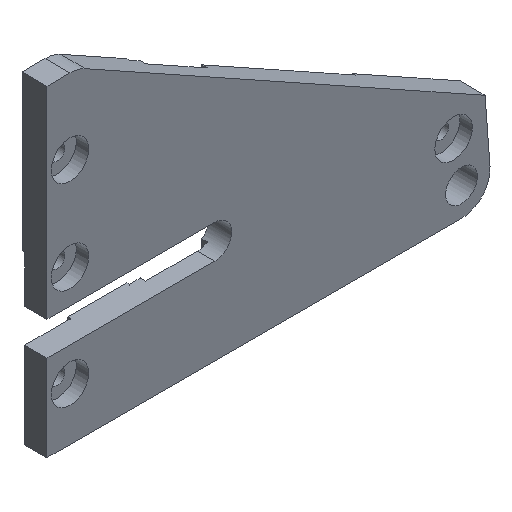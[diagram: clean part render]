
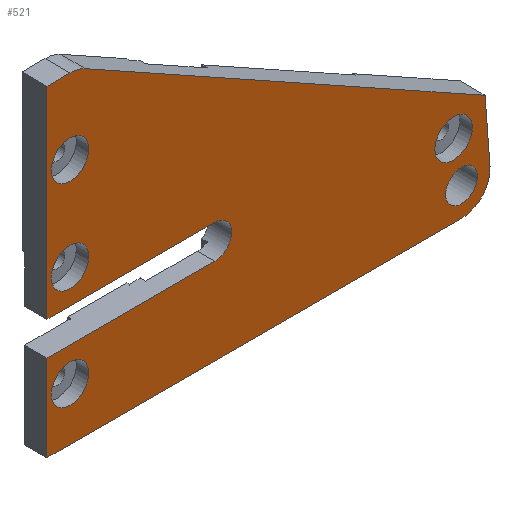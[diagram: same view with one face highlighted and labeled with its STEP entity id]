
A CAD part, isometric view. The second image highlights one B-rep face of the part: STEP entity #521.
In plain terms, the highlighted planar face has unit normal (0, -1, 0).
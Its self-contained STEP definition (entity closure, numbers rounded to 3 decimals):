
#18 = ORIENTED_EDGE ( 'NONE', *, *, #1301, .T. ) ;
#49 = EDGE_CURVE ( 'NONE', #352, #352, #270, .T. ) ;
#84 = EDGE_CURVE ( 'NONE', #267, #700, #531, .T. ) ;
#111 = CARTESIAN_POINT ( 'NONE',  ( 4.597, -5., -33.63 ) ) ;
#112 = EDGE_LOOP ( 'NONE', ( #823 ) ) ;
#125 = ORIENTED_EDGE ( 'NONE', *, *, #84, .T. ) ;
#140 = DIRECTION ( 'NONE',  ( 0., -1., 0. ) ) ;
#162 = CARTESIAN_POINT ( 'NONE',  ( 0., -5., 0. ) ) ;
#174 = FACE_BOUND ( 'NONE', #292, .T. ) ;
#187 = LINE ( 'NONE', #744, #439 ) ;
#190 = VECTOR ( 'NONE', #1303, 1000. ) ;
#191 = VERTEX_POINT ( 'NONE', #162 ) ;
#199 = CARTESIAN_POINT ( 'NONE',  ( 4.597, -5., -57.573 ) ) ;
#203 = VERTEX_POINT ( 'NONE', #1128 ) ;
#210 = CARTESIAN_POINT ( 'NONE',  ( 33.579, -5., -43.726 ) ) ;
#220 = DIRECTION ( 'NONE',  ( 0., 0., -1. ) ) ;
#244 = ORIENTED_EDGE ( 'NONE', *, *, #445, .T. ) ;
#247 = ORIENTED_EDGE ( 'NONE', *, *, #398, .F. ) ;
#254 = VERTEX_POINT ( 'NONE', #737 ) ;
#258 = CARTESIAN_POINT ( 'NONE',  ( 81.344, -5., -49.72 ) ) ;
#260 = LINE ( 'NONE', #1119, #1366 ) ;
#267 = VERTEX_POINT ( 'NONE', #607 ) ;
#270 = CIRCLE ( 'NONE', #540, 3.75 ) ;
#279 = EDGE_CURVE ( 'NONE', #687, #1189, #896, .T. ) ;
#289 = VERTEX_POINT ( 'NONE', #1157 ) ;
#292 = EDGE_LOOP ( 'NONE', ( #1288 ) ) ;
#303 = CARTESIAN_POINT ( 'NONE',  ( 82.931, -5., -55.474 ) ) ;
#317 = AXIS2_PLACEMENT_3D ( 'NONE', #1224, #589, #1336 ) ;
#320 = DIRECTION ( 'NONE',  ( 0., 0., 1. ) ) ;
#324 = EDGE_CURVE ( 'NONE', #1141, #1141, #838, .T. ) ;
#328 = CARTESIAN_POINT ( 'NONE',  ( 0., -5., 0. ) ) ;
#330 = LINE ( 'NONE', #328, #1144 ) ;
#337 = AXIS2_PLACEMENT_3D ( 'NONE', #983, #345, #1096 ) ;
#343 = CIRCLE ( 'NONE', #1369, 3.366 ) ;
#345 = DIRECTION ( 'NONE',  ( 0., -1., 0. ) ) ;
#352 = VERTEX_POINT ( 'NONE', #622 ) ;
#355 = DIRECTION ( 'NONE',  ( 0., 1., 0. ) ) ;
#357 = CIRCLE ( 'NONE', #966, 3.75 ) ;
#359 = AXIS2_PLACEMENT_3D ( 'NONE', #614, #1357, #721 ) ;
#361 = DIRECTION ( 'NONE',  ( 0., 0., -1. ) ) ;
#384 = CARTESIAN_POINT ( 'NONE',  ( 1.482, -5., 2.657 ) ) ;
#391 = DIRECTION ( 'NONE',  ( 1., 0., 0. ) ) ;
#398 = EDGE_CURVE ( 'NONE', #584, #203, #343, .T. ) ;
#402 = ORIENTED_EDGE ( 'NONE', *, *, #279, .T. ) ;
#415 = LINE ( 'NONE', #613, #947 ) ;
#426 = LINE ( 'NONE', #1245, #1237 ) ;
#427 = VERTEX_POINT ( 'NONE', #1196 ) ;
#432 = DIRECTION ( 'NONE',  ( 0., 0., -1. ) ) ;
#439 = VECTOR ( 'NONE', #1058, 1000. ) ;
#445 = EDGE_CURVE ( 'NONE', #700, #1307, #565, .T. ) ;
#455 = EDGE_LOOP ( 'NONE', ( #711 ) ) ;
#457 = CARTESIAN_POINT ( 'NONE',  ( 0., -5., 0. ) ) ;
#459 = FACE_BOUND ( 'NONE', #112, .T. ) ;
#474 = LINE ( 'NONE', #1193, #190 ) ;
#496 = DIRECTION ( 'NONE',  ( -0.873, 0., 0.487 ) ) ;
#514 = ORIENTED_EDGE ( 'NONE', *, *, #761, .F. ) ;
#521 = ADVANCED_FACE ( 'NONE', ( #459, #1311, #174, #1282, #991, #715 ), #992, .F. ) ;
#531 = LINE ( 'NONE', #900, #1025 ) ;
#540 = AXIS2_PLACEMENT_3D ( 'NONE', #787, #140, #894 ) ;
#565 = CIRCLE ( 'NONE', #337, 5.715 ) ;
#581 = CARTESIAN_POINT ( 'NONE',  ( 4.597, -5., 0. ) ) ;
#582 = EDGE_CURVE ( 'NONE', #289, #289, #357, .T. ) ;
#584 = VERTEX_POINT ( 'NONE', #791 ) ;
#589 = DIRECTION ( 'NONE',  ( 0., -1., 0. ) ) ;
#607 = CARTESIAN_POINT ( 'NONE',  ( 0., -5., -64.364 ) ) ;
#613 = CARTESIAN_POINT ( 'NONE',  ( 0., -5., -47.092 ) ) ;
#614 = CARTESIAN_POINT ( 'NONE',  ( 4.597, -5., -6.35 ) ) ;
#622 = CARTESIAN_POINT ( 'NONE',  ( 4.597, -5., -18.75 ) ) ;
#625 = CARTESIAN_POINT ( 'NONE',  ( 82.931, -5., -58.649 ) ) ;
#644 = EDGE_CURVE ( 'NONE', #191, #1189, #260, .T. ) ;
#653 = AXIS2_PLACEMENT_3D ( 'NONE', #625, #1370, #735 ) ;
#685 = DIRECTION ( 'NONE',  ( 1., 0., 0. ) ) ;
#687 = VERTEX_POINT ( 'NONE', #1343 ) ;
#700 = VERTEX_POINT ( 'NONE', #1127 ) ;
#711 = ORIENTED_EDGE ( 'NONE', *, *, #1235, .F. ) ;
#715 = FACE_OUTER_BOUND ( 'NONE', #745, .T. ) ;
#721 = DIRECTION ( 'NONE',  ( 0., 0., -1. ) ) ;
#735 = DIRECTION ( 'NONE',  ( 0., 0., 1. ) ) ;
#737 = CARTESIAN_POINT ( 'NONE',  ( 4.597, -5., -37.38 ) ) ;
#744 = CARTESIAN_POINT ( 'NONE',  ( 83.678, -5., 6.412 ) ) ;
#745 = EDGE_LOOP ( 'NONE', ( #402, #1186, #1165, #1176, #247, #514, #905, #125, #244, #1361, #18 ) ) ;
#761 = EDGE_CURVE ( 'NONE', #427, #584, #415, .T. ) ;
#787 = CARTESIAN_POINT ( 'NONE',  ( 4.597, -5., -15. ) ) ;
#789 = VERTEX_POINT ( 'NONE', #199 ) ;
#791 = CARTESIAN_POINT ( 'NONE',  ( 33.579, -5., -47.092 ) ) ;
#810 = LINE ( 'NONE', #384, #1344 ) ;
#823 = ORIENTED_EDGE ( 'NONE', *, *, #324, .T. ) ;
#838 = CIRCLE ( 'NONE', #653, 3.175 ) ;
#865 = DIRECTION ( 'NONE',  ( 0., -1., 0. ) ) ;
#873 = EDGE_CURVE ( 'NONE', #972, #1307, #187, .T. ) ;
#877 = CIRCLE ( 'NONE', #317, 3.75 ) ;
#893 = AXIS2_PLACEMENT_3D ( 'NONE', #457, #355, #1103 ) ;
#894 = DIRECTION ( 'NONE',  ( 0., 0., -1. ) ) ;
#896 = CIRCLE ( 'NONE', #359, 6.35 ) ;
#900 = CARTESIAN_POINT ( 'NONE',  ( 0., -5., -64.364 ) ) ;
#901 = ORIENTED_EDGE ( 'NONE', *, *, #582, .F. ) ;
#905 = ORIENTED_EDGE ( 'NONE', *, *, #1116, .T. ) ;
#906 = DIRECTION ( 'NONE',  ( 1., 0., 0. ) ) ;
#947 = VECTOR ( 'NONE', #391, 1000. ) ;
#956 = DIRECTION ( 'NONE',  ( 0., -1., 0. ) ) ;
#966 = AXIS2_PLACEMENT_3D ( 'NONE', #258, #1001, #361 ) ;
#972 = VERTEX_POINT ( 'NONE', #1283 ) ;
#983 = CARTESIAN_POINT ( 'NONE',  ( 82.931, -5., -58.649 ) ) ;
#991 = FACE_BOUND ( 'NONE', #455, .T. ) ;
#992 = PLANE ( 'NONE',  #893 ) ;
#994 = EDGE_CURVE ( 'NONE', #191, #1289, #330, .T. ) ;
#1001 = DIRECTION ( 'NONE',  ( 0., -1., 0. ) ) ;
#1010 = EDGE_CURVE ( 'NONE', #254, #254, #1180, .T. ) ;
#1025 = VECTOR ( 'NONE', #685, 1000. ) ;
#1040 = DIRECTION ( 'NONE',  ( -1., 0., 0. ) ) ;
#1049 = ORIENTED_EDGE ( 'NONE', *, *, #49, .F. ) ;
#1058 = DIRECTION ( 'NONE',  ( 0.076, 0., -0.997 ) ) ;
#1096 = DIRECTION ( 'NONE',  ( 0., 0., 1. ) ) ;
#1103 = DIRECTION ( 'NONE',  ( 0., 0., 1. ) ) ;
#1116 = EDGE_CURVE ( 'NONE', #427, #267, #474, .T. ) ;
#1119 = CARTESIAN_POINT ( 'NONE',  ( 0., -5., 0. ) ) ;
#1127 = CARTESIAN_POINT ( 'NONE',  ( 82.931, -5., -64.364 ) ) ;
#1128 = CARTESIAN_POINT ( 'NONE',  ( 33.579, -5., -40.361 ) ) ;
#1133 = CARTESIAN_POINT ( 'NONE',  ( 88.629, -5., -58.212 ) ) ;
#1141 = VERTEX_POINT ( 'NONE', #303 ) ;
#1144 = VECTOR ( 'NONE', #432, 1000. ) ;
#1157 = CARTESIAN_POINT ( 'NONE',  ( 81.344, -5., -53.47 ) ) ;
#1165 = ORIENTED_EDGE ( 'NONE', *, *, #994, .T. ) ;
#1176 = ORIENTED_EDGE ( 'NONE', *, *, #1355, .F. ) ;
#1180 = CIRCLE ( 'NONE', #1371, 3.75 ) ;
#1186 = ORIENTED_EDGE ( 'NONE', *, *, #644, .F. ) ;
#1189 = VERTEX_POINT ( 'NONE', #581 ) ;
#1193 = CARTESIAN_POINT ( 'NONE',  ( 0., -5., 0. ) ) ;
#1196 = CARTESIAN_POINT ( 'NONE',  ( 0., -5., -47.092 ) ) ;
#1224 = CARTESIAN_POINT ( 'NONE',  ( 4.597, -5., -53.823 ) ) ;
#1233 = CARTESIAN_POINT ( 'NONE',  ( 0., -5., -40.361 ) ) ;
#1235 = EDGE_CURVE ( 'NONE', #789, #789, #877, .T. ) ;
#1237 = VECTOR ( 'NONE', #1040, 1000. ) ;
#1245 = CARTESIAN_POINT ( 'NONE',  ( 0., -5., -40.361 ) ) ;
#1282 = FACE_BOUND ( 'NONE', #1395, .T. ) ;
#1283 = CARTESIAN_POINT ( 'NONE',  ( 87.647, -5., -45.387 ) ) ;
#1288 = ORIENTED_EDGE ( 'NONE', *, *, #1010, .F. ) ;
#1289 = VERTEX_POINT ( 'NONE', #1233 ) ;
#1300 = EDGE_LOOP ( 'NONE', ( #901 ) ) ;
#1301 = EDGE_CURVE ( 'NONE', #972, #687, #810, .T. ) ;
#1303 = DIRECTION ( 'NONE',  ( 0., 0., -1. ) ) ;
#1307 = VERTEX_POINT ( 'NONE', #1133 ) ;
#1311 = FACE_BOUND ( 'NONE', #1300, .T. ) ;
#1336 = DIRECTION ( 'NONE',  ( 0., 0., -1. ) ) ;
#1343 = CARTESIAN_POINT ( 'NONE',  ( 7.689, -5., -0.804 ) ) ;
#1344 = VECTOR ( 'NONE', #496, 1000. ) ;
#1355 = EDGE_CURVE ( 'NONE', #203, #1289, #426, .T. ) ;
#1357 = DIRECTION ( 'NONE',  ( 0., -1., 0. ) ) ;
#1361 = ORIENTED_EDGE ( 'NONE', *, *, #873, .F. ) ;
#1366 = VECTOR ( 'NONE', #906, 1000. ) ;
#1369 = AXIS2_PLACEMENT_3D ( 'NONE', #210, #956, #320 ) ;
#1370 = DIRECTION ( 'NONE',  ( 0., 1., 0. ) ) ;
#1371 = AXIS2_PLACEMENT_3D ( 'NONE', #111, #865, #220 ) ;
#1395 = EDGE_LOOP ( 'NONE', ( #1049 ) ) ;
